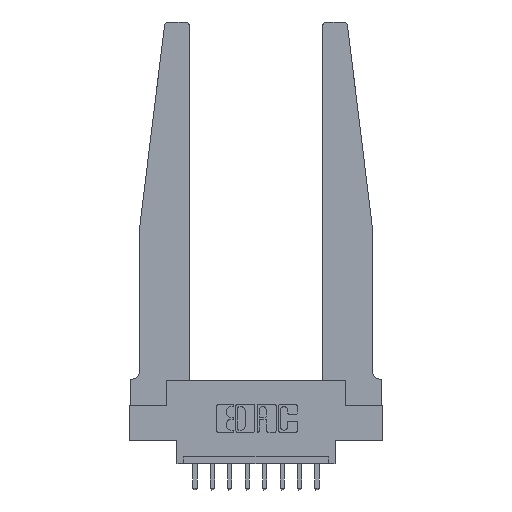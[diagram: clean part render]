
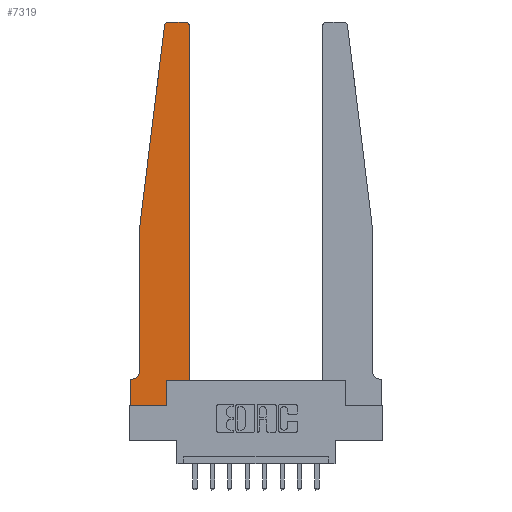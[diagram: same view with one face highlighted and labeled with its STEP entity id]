
A CAD part, top view. The second image highlights one B-rep face of the part: STEP entity #7319.
In plain terms, the highlighted planar face has unit normal (0, 0, 1).
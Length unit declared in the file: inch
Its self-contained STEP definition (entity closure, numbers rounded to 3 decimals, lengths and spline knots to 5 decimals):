
#25 = VERTEX_POINT ( 'NONE', #9697 ) ;
#51 = CARTESIAN_POINT ( 'NONE',  ( 0.24675, 2.72367, 0.37 ) ) ;
#181 = VERTEX_POINT ( 'NONE', #2225 ) ;
#333 = LINE ( 'NONE', #978, #7143 ) ;
#363 = ORIENTED_EDGE ( 'NONE', *, *, #8477, .T. ) ;
#368 = EDGE_CURVE ( 'NONE', #181, #14049, #333, .T. ) ;
#520 = LINE ( 'NONE', #5339, #870 ) ;
#687 = FACE_OUTER_BOUND ( 'NONE', #13571, .T. ) ;
#745 = ORIENTED_EDGE ( 'NONE', *, *, #6395, .T. ) ;
#764 = EDGE_CURVE ( 'NONE', #3584, #4420, #10306, .T. ) ;
#831 = AXIS2_PLACEMENT_3D ( 'NONE', #5121, #14120, #9660 ) ;
#870 = VECTOR ( 'NONE', #13237, 39.37008 ) ;
#922 = ORIENTED_EDGE ( 'NONE', *, *, #368, .T. ) ;
#978 = CARTESIAN_POINT ( 'NONE',  ( 0.25, 2.75, 0.37 ) ) ;
#1075 = VERTEX_POINT ( 'NONE', #1097 ) ;
#1097 = CARTESIAN_POINT ( 'NONE',  ( 0.425, 2.72, 0.37 ) ) ;
#1128 = ORIENTED_EDGE ( 'NONE', *, *, #7257, .T. ) ;
#1243 = DIRECTION ( 'NONE',  ( 0., 1., 0. ) ) ;
#1362 = CARTESIAN_POINT ( 'NONE',  ( 0., 0.1875, 0.37 ) ) ;
#1396 = CARTESIAN_POINT ( 'NONE',  ( 0.425, 0.18, 0.37 ) ) ;
#1648 = DIRECTION ( 'NONE',  ( 1., 0., 0. ) ) ;
#2055 = DIRECTION ( 'NONE',  ( -0.122, -0.992, 0. ) ) ;
#2225 = CARTESIAN_POINT ( 'NONE',  ( 0.395, 2.75, 0.37 ) ) ;
#2455 = ORIENTED_EDGE ( 'NONE', *, *, #8939, .T. ) ;
#2631 = CIRCLE ( 'NONE', #831, 0.05 ) ;
#3001 = CARTESIAN_POINT ( 'NONE',  ( 0.395, 2.72, 0.37 ) ) ;
#3033 = ORIENTED_EDGE ( 'NONE', *, *, #5741, .T. ) ;
#3062 = CARTESIAN_POINT ( 'NONE',  ( 0., 0.1875, 0.37 ) ) ;
#3106 = DIRECTION ( 'NONE',  ( 0., 0., 1. ) ) ;
#3584 = VERTEX_POINT ( 'NONE', #51 ) ;
#3585 = DIRECTION ( 'NONE',  ( 0., 1., 0. ) ) ;
#3724 = LINE ( 'NONE', #7434, #13000 ) ;
#3744 = AXIS2_PLACEMENT_3D ( 'NONE', #3001, #3106, #5262 ) ;
#4095 = CIRCLE ( 'NONE', #3744, 0.03 ) ;
#4412 = EDGE_CURVE ( 'NONE', #10425, #25, #12328, .T. ) ;
#4420 = VERTEX_POINT ( 'NONE', #13814 ) ;
#5121 = CARTESIAN_POINT ( 'NONE',  ( 0.015, 0.2375, 0.37 ) ) ;
#5262 = DIRECTION ( 'NONE',  ( 1., 0., 0. ) ) ;
#5339 = CARTESIAN_POINT ( 'NONE',  ( 0.065, 0.1875, 0.37 ) ) ;
#5421 = PLANE ( 'NONE',  #12859 ) ;
#5496 = VECTOR ( 'NONE', #12731, 39.37008 ) ;
#5741 = EDGE_CURVE ( 'NONE', #1075, #181, #4095, .T. ) ;
#5772 = VERTEX_POINT ( 'NONE', #8118 ) ;
#6069 = CIRCLE ( 'NONE', #9604, 0.03 ) ;
#6338 = DIRECTION ( 'NONE',  ( -1., 0., 0. ) ) ;
#6395 = EDGE_CURVE ( 'NONE', #5772, #13739, #3724, .T. ) ;
#6541 = DIRECTION ( 'NONE',  ( 0., 0., 1. ) ) ;
#6933 = VECTOR ( 'NONE', #3585, 39.37008 ) ;
#6953 = VERTEX_POINT ( 'NONE', #12606 ) ;
#7025 = CARTESIAN_POINT ( 'NONE',  ( 0.27653, 2.75, 0.37 ) ) ;
#7143 = VECTOR ( 'NONE', #6338, 39.37008 ) ;
#7257 = EDGE_CURVE ( 'NONE', #6953, #7506, #2631, .T. ) ;
#7319 = ADVANCED_FACE ( 'NONE', ( #687 ), #5421, .T. ) ;
#7434 = CARTESIAN_POINT ( 'NONE',  ( 0., 0., 0.37 ) ) ;
#7498 = VERTEX_POINT ( 'NONE', #1362 ) ;
#7506 = VERTEX_POINT ( 'NONE', #12589 ) ;
#8118 = CARTESIAN_POINT ( 'NONE',  ( 0., 0., 0.37 ) ) ;
#8477 = EDGE_CURVE ( 'NONE', #7498, #5772, #9056, .T. ) ;
#8682 = LINE ( 'NONE', #14407, #10468 ) ;
#8778 = DIRECTION ( 'NONE',  ( 1., 0., 0. ) ) ;
#8887 = CARTESIAN_POINT ( 'NONE',  ( 0., 0., 0.37 ) ) ;
#8933 = CARTESIAN_POINT ( 'NONE',  ( 0.27653, 2.72, 0.37 ) ) ;
#8939 = EDGE_CURVE ( 'NONE', #13739, #10425, #8682, .T. ) ;
#9056 = LINE ( 'NONE', #8887, #13118 ) ;
#9136 = DIRECTION ( 'NONE',  ( 0., -1., 0. ) ) ;
#9604 = AXIS2_PLACEMENT_3D ( 'NONE', #8933, #6541, #14436 ) ;
#9660 = DIRECTION ( 'NONE',  ( -1., 0., 0. ) ) ;
#9697 = CARTESIAN_POINT ( 'NONE',  ( 0.425, 0.18, 0.37 ) ) ;
#9865 = ORIENTED_EDGE ( 'NONE', *, *, #10405, .T. ) ;
#10254 = CARTESIAN_POINT ( 'NONE',  ( 0.065, 1.25, 0.37 ) ) ;
#10306 = LINE ( 'NONE', #10254, #10998 ) ;
#10339 = VECTOR ( 'NONE', #14506, 39.37008 ) ;
#10405 = EDGE_CURVE ( 'NONE', #25, #1075, #13093, .T. ) ;
#10425 = VERTEX_POINT ( 'NONE', #11508 ) ;
#10468 = VECTOR ( 'NONE', #1243, 39.37008 ) ;
#10602 = CARTESIAN_POINT ( 'NONE',  ( 0.2605, 0., 0.37 ) ) ;
#10715 = EDGE_CURVE ( 'NONE', #14049, #3584, #6069, .T. ) ;
#10856 = LINE ( 'NONE', #13403, #10339 ) ;
#10998 = VECTOR ( 'NONE', #2055, 39.37008 ) ;
#11029 = ORIENTED_EDGE ( 'NONE', *, *, #764, .T. ) ;
#11113 = ORIENTED_EDGE ( 'NONE', *, *, #4412, .T. ) ;
#11410 = CARTESIAN_POINT ( 'NONE',  ( 0.425, 0.18, 0.37 ) ) ;
#11508 = CARTESIAN_POINT ( 'NONE',  ( 0.2605, 0.18, 0.37 ) ) ;
#11675 = ORIENTED_EDGE ( 'NONE', *, *, #12630, .T. ) ;
#12193 = DIRECTION ( 'NONE',  ( 0., 0., 1. ) ) ;
#12328 = LINE ( 'NONE', #1396, #5496 ) ;
#12589 = CARTESIAN_POINT ( 'NONE',  ( 0.015, 0.1875, 0.37 ) ) ;
#12606 = CARTESIAN_POINT ( 'NONE',  ( 0.065, 0.2375, 0.37 ) ) ;
#12630 = EDGE_CURVE ( 'NONE', #4420, #6953, #10856, .T. ) ;
#12731 = DIRECTION ( 'NONE',  ( 1., 0., 0. ) ) ;
#12859 = AXIS2_PLACEMENT_3D ( 'NONE', #3062, #12193, #8778 ) ;
#13000 = VECTOR ( 'NONE', #1648, 39.37008 ) ;
#13093 = LINE ( 'NONE', #11410, #6933 ) ;
#13118 = VECTOR ( 'NONE', #9136, 39.37008 ) ;
#13153 = EDGE_CURVE ( 'NONE', #7506, #7498, #520, .T. ) ;
#13237 = DIRECTION ( 'NONE',  ( -1., 0., 0. ) ) ;
#13403 = CARTESIAN_POINT ( 'NONE',  ( 0.065, 1.25, 0.37 ) ) ;
#13521 = ORIENTED_EDGE ( 'NONE', *, *, #13153, .T. ) ;
#13571 = EDGE_LOOP ( 'NONE', ( #922, #14233, #11029, #11675, #1128, #13521, #363, #745, #2455, #11113, #9865, #3033 ) ) ;
#13739 = VERTEX_POINT ( 'NONE', #10602 ) ;
#13814 = CARTESIAN_POINT ( 'NONE',  ( 0.065, 1.25, 0.37 ) ) ;
#14049 = VERTEX_POINT ( 'NONE', #7025 ) ;
#14120 = DIRECTION ( 'NONE',  ( 0., 0., -1. ) ) ;
#14233 = ORIENTED_EDGE ( 'NONE', *, *, #10715, .T. ) ;
#14407 = CARTESIAN_POINT ( 'NONE',  ( 0.2605, 0.18, 0.37 ) ) ;
#14436 = DIRECTION ( 'NONE',  ( 1., 0., 0. ) ) ;
#14506 = DIRECTION ( 'NONE',  ( 0., -1., 0. ) ) ;
